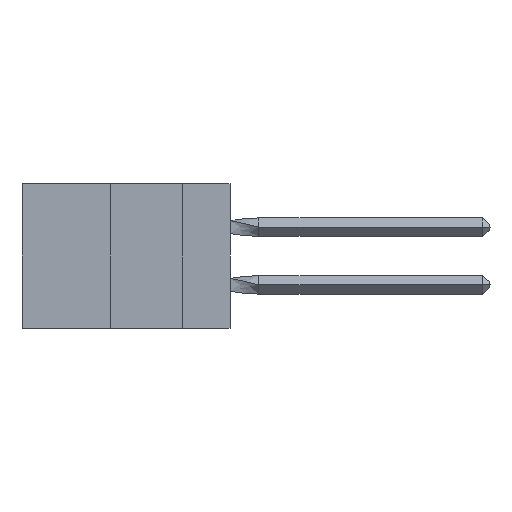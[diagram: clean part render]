
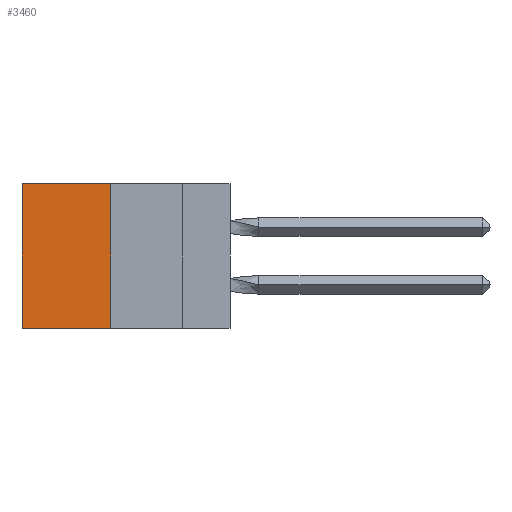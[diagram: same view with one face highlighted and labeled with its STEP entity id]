
A CAD part, left-side view. The second image highlights one B-rep face of the part: STEP entity #3460.
In plain terms, the highlighted planar face has unit normal (-1, 0, 0).
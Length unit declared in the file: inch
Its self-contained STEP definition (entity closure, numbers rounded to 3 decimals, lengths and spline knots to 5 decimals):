
#1232 = VECTOR ( 'NONE', #2807, 39.37008 ) ;
#1393 = DIRECTION ( 'NONE',  ( 0., 1., 0. ) ) ;
#1451 = VECTOR ( 'NONE', #11924, 39.37008 ) ;
#1513 = DIRECTION ( 'NONE',  ( 0., 0., -1. ) ) ;
#2246 = LINE ( 'NONE', #20153, #1451 ) ;
#2807 = DIRECTION ( 'NONE',  ( 0., 0., -1. ) ) ;
#3107 = CARTESIAN_POINT ( 'NONE',  ( 0.305, 0.413, -0.5 ) ) ;
#3460 = ADVANCED_FACE ( 'NONE', ( #5463 ), #18084, .F. ) ;
#3952 = EDGE_CURVE ( 'NONE', #16363, #10835, #6444, .T. ) ;
#4017 = EDGE_CURVE ( 'NONE', #10835, #12089, #2246, .T. ) ;
#4860 = CARTESIAN_POINT ( 'NONE',  ( 0.305, 0.413, -0.5 ) ) ;
#5463 = FACE_OUTER_BOUND ( 'NONE', #13469, .T. ) ;
#5892 = VERTEX_POINT ( 'NONE', #3107 ) ;
#6141 = VECTOR ( 'NONE', #10403, 39.37008 ) ;
#6444 = LINE ( 'NONE', #19786, #10337 ) ;
#6969 = CARTESIAN_POINT ( 'NONE',  ( 0.305, 0.413, 0. ) ) ;
#7006 = LINE ( 'NONE', #9321, #1232 ) ;
#7488 = ORIENTED_EDGE ( 'NONE', *, *, #3952, .T. ) ;
#8668 = CARTESIAN_POINT ( 'NONE',  ( 0.305, 0.413, -0.5 ) ) ;
#9281 = CARTESIAN_POINT ( 'NONE',  ( 0.305, 0.72, -0.5 ) ) ;
#9321 = CARTESIAN_POINT ( 'NONE',  ( 0.305, 0.413, -0.5 ) ) ;
#10141 = AXIS2_PLACEMENT_3D ( 'NONE', #4860, #18161, #1513 ) ;
#10324 = EDGE_CURVE ( 'NONE', #16363, #5892, #7006, .T. ) ;
#10337 = VECTOR ( 'NONE', #1393, 39.37008 ) ;
#10403 = DIRECTION ( 'NONE',  ( 0., 1., 0. ) ) ;
#10835 = VERTEX_POINT ( 'NONE', #16131 ) ;
#11924 = DIRECTION ( 'NONE',  ( 0., 0., -1. ) ) ;
#12033 = ORIENTED_EDGE ( 'NONE', *, *, #10324, .F. ) ;
#12089 = VERTEX_POINT ( 'NONE', #9281 ) ;
#13469 = EDGE_LOOP ( 'NONE', ( #20359, #21513, #12033, #7488 ) ) ;
#16131 = CARTESIAN_POINT ( 'NONE',  ( 0.305, 0.72, 0. ) ) ;
#16363 = VERTEX_POINT ( 'NONE', #6969 ) ;
#18084 = PLANE ( 'NONE',  #10141 ) ;
#18161 = DIRECTION ( 'NONE',  ( 1., 0., 0. ) ) ;
#18227 = EDGE_CURVE ( 'NONE', #5892, #12089, #18844, .T. ) ;
#18844 = LINE ( 'NONE', #8668, #6141 ) ;
#19786 = CARTESIAN_POINT ( 'NONE',  ( 0.305, 0.413, 0. ) ) ;
#20153 = CARTESIAN_POINT ( 'NONE',  ( 0.305, 0.72, -0.5 ) ) ;
#20359 = ORIENTED_EDGE ( 'NONE', *, *, #4017, .T. ) ;
#21513 = ORIENTED_EDGE ( 'NONE', *, *, #18227, .F. ) ;
